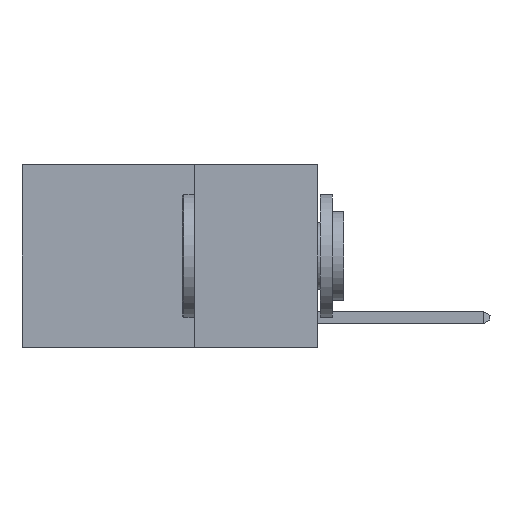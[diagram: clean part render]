
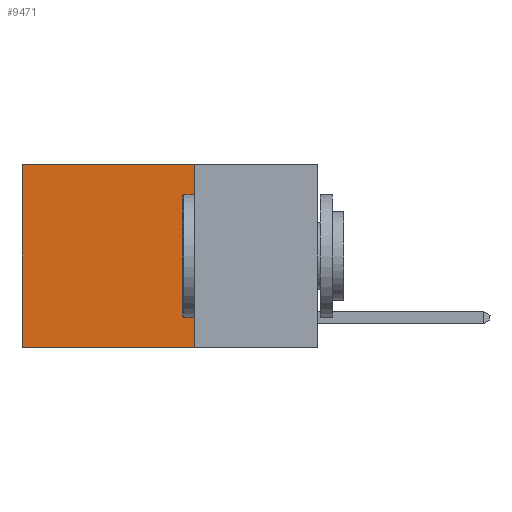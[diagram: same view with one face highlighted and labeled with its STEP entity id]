
A CAD part, left-side view. The second image highlights one B-rep face of the part: STEP entity #9471.
In plain terms, the highlighted planar face has unit normal (-1, 0, 0).
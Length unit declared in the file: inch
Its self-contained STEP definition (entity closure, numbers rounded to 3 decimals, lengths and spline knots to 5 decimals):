
#9 = AXIS2_PLACEMENT_3D ( 'NONE', #10530, #4483, #9549 ) ;
#162 = ORIENTED_EDGE ( 'NONE', *, *, #1094, .T. ) ;
#1094 = EDGE_CURVE ( 'NONE', #10960, #2678, #4581, .T. ) ;
#1101 = CARTESIAN_POINT ( 'NONE',  ( 0.2625, 0.25, -0.37 ) ) ;
#1869 = CARTESIAN_POINT ( 'NONE',  ( 0.2625, 0.25, 0. ) ) ;
#1968 = VECTOR ( 'NONE', #2839, 39.37008 ) ;
#2678 = VERTEX_POINT ( 'NONE', #8848 ) ;
#2839 = DIRECTION ( 'NONE',  ( 0., 0., -1. ) ) ;
#3641 = FACE_OUTER_BOUND ( 'NONE', #7669, .T. ) ;
#3661 = VECTOR ( 'NONE', #7889, 39.37008 ) ;
#3697 = PLANE ( 'NONE',  #9 ) ;
#3898 = LINE ( 'NONE', #9012, #4344 ) ;
#4338 = LINE ( 'NONE', #1869, #3661 ) ;
#4344 = VECTOR ( 'NONE', #7355, 39.37008 ) ;
#4483 = DIRECTION ( 'NONE',  ( 1., 0., 0. ) ) ;
#4581 = LINE ( 'NONE', #7180, #1968 ) ;
#5631 = EDGE_CURVE ( 'NONE', #9198, #10960, #3898, .T. ) ;
#5663 = CARTESIAN_POINT ( 'NONE',  ( 0.2625, 0.25, 0. ) ) ;
#6226 = VERTEX_POINT ( 'NONE', #9309 ) ;
#6419 = ORIENTED_EDGE ( 'NONE', *, *, #5631, .T. ) ;
#7180 = CARTESIAN_POINT ( 'NONE',  ( 0.2625, 0.6, 0. ) ) ;
#7280 = EDGE_CURVE ( 'NONE', #6226, #2678, #9715, .T. ) ;
#7355 = DIRECTION ( 'NONE',  ( 0., 1., 0. ) ) ;
#7483 = ORIENTED_EDGE ( 'NONE', *, *, #7280, .F. ) ;
#7669 = EDGE_LOOP ( 'NONE', ( #162, #7483, #9564, #6419 ) ) ;
#7889 = DIRECTION ( 'NONE',  ( 0., 0., -1. ) ) ;
#7931 = VECTOR ( 'NONE', #10624, 39.37008 ) ;
#8848 = CARTESIAN_POINT ( 'NONE',  ( 0.2625, 0.6, -0.37 ) ) ;
#9012 = CARTESIAN_POINT ( 'NONE',  ( 0.2625, 0.25, 0. ) ) ;
#9198 = VERTEX_POINT ( 'NONE', #5663 ) ;
#9309 = CARTESIAN_POINT ( 'NONE',  ( 0.2625, 0.25, -0.37 ) ) ;
#9471 = ADVANCED_FACE ( 'NONE', ( #3641 ), #3697, .F. ) ;
#9549 = DIRECTION ( 'NONE',  ( 0., 0., -1. ) ) ;
#9564 = ORIENTED_EDGE ( 'NONE', *, *, #10249, .F. ) ;
#9715 = LINE ( 'NONE', #1101, #7931 ) ;
#9793 = CARTESIAN_POINT ( 'NONE',  ( 0.2625, 0.6, 0. ) ) ;
#10249 = EDGE_CURVE ( 'NONE', #9198, #6226, #4338, .T. ) ;
#10530 = CARTESIAN_POINT ( 'NONE',  ( 0.2625, 0.25, 0. ) ) ;
#10624 = DIRECTION ( 'NONE',  ( 0., 1., 0. ) ) ;
#10960 = VERTEX_POINT ( 'NONE', #9793 ) ;
